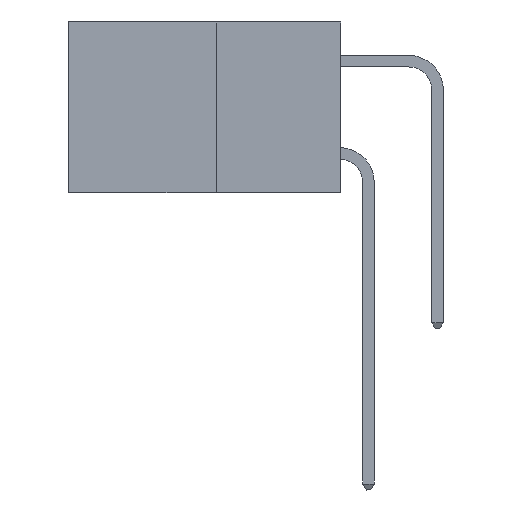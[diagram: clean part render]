
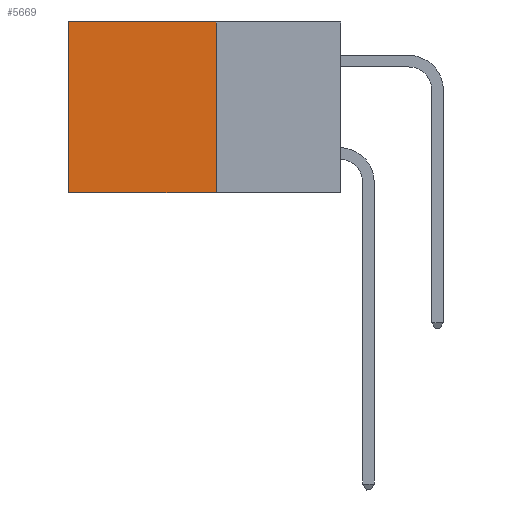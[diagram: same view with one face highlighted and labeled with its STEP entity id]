
A CAD part, left-side view. The second image highlights one B-rep face of the part: STEP entity #5669.
In plain terms, the highlighted planar face has unit normal (-1, 0, 0).
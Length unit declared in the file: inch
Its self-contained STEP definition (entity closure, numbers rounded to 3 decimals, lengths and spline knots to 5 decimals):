
#423 = EDGE_CURVE ( 'NONE', #3450, #9544, #16978, .T. ) ;
#1078 = DIRECTION ( 'NONE',  ( 0., 1., 0. ) ) ;
#1513 = EDGE_CURVE ( 'NONE', #9544, #7395, #6821, .T. ) ;
#2710 = VECTOR ( 'NONE', #7247, 39.37008 ) ;
#3160 = LINE ( 'NONE', #5839, #2710 ) ;
#3450 = VERTEX_POINT ( 'NONE', #7370 ) ;
#3506 = VECTOR ( 'NONE', #7274, 39.37008 ) ;
#4459 = CARTESIAN_POINT ( 'NONE',  ( 0.277, 0.27, -0.37 ) ) ;
#5669 = ADVANCED_FACE ( 'NONE', ( #13820 ), #6727, .F. ) ;
#5753 = VECTOR ( 'NONE', #17899, 39.37008 ) ;
#5764 = CARTESIAN_POINT ( 'NONE',  ( 0.277, 0.59, 0. ) ) ;
#5839 = CARTESIAN_POINT ( 'NONE',  ( 0.277, 0.27, -0.37 ) ) ;
#6727 = PLANE ( 'NONE',  #17481 ) ;
#6821 = LINE ( 'NONE', #13843, #3506 ) ;
#7247 = DIRECTION ( 'NONE',  ( 0., 0., -1. ) ) ;
#7274 = DIRECTION ( 'NONE',  ( 0., 0., -1. ) ) ;
#7370 = CARTESIAN_POINT ( 'NONE',  ( 0.277, 0.27, 0. ) ) ;
#7395 = VERTEX_POINT ( 'NONE', #14229 ) ;
#8131 = DIRECTION ( 'NONE',  ( 1., 0., 0. ) ) ;
#8207 = EDGE_CURVE ( 'NONE', #16064, #7395, #10710, .T. ) ;
#9095 = EDGE_LOOP ( 'NONE', ( #12071, #12832, #16765, #14040 ) ) ;
#9544 = VERTEX_POINT ( 'NONE', #5764 ) ;
#10710 = LINE ( 'NONE', #16566, #5753 ) ;
#12071 = ORIENTED_EDGE ( 'NONE', *, *, #1513, .T. ) ;
#12170 = EDGE_CURVE ( 'NONE', #3450, #16064, #3160, .T. ) ;
#12323 = CARTESIAN_POINT ( 'NONE',  ( 0.277, 0.27, 0. ) ) ;
#12832 = ORIENTED_EDGE ( 'NONE', *, *, #8207, .F. ) ;
#13820 = FACE_OUTER_BOUND ( 'NONE', #9095, .T. ) ;
#13843 = CARTESIAN_POINT ( 'NONE',  ( 0.277, 0.59, -0.37 ) ) ;
#14040 = ORIENTED_EDGE ( 'NONE', *, *, #423, .T. ) ;
#14229 = CARTESIAN_POINT ( 'NONE',  ( 0.277, 0.59, -0.37 ) ) ;
#16064 = VERTEX_POINT ( 'NONE', #4459 ) ;
#16335 = CARTESIAN_POINT ( 'NONE',  ( 0.277, 0.27, -0.37 ) ) ;
#16566 = CARTESIAN_POINT ( 'NONE',  ( 0.277, 0.27, -0.37 ) ) ;
#16580 = VECTOR ( 'NONE', #1078, 39.37008 ) ;
#16765 = ORIENTED_EDGE ( 'NONE', *, *, #12170, .F. ) ;
#16978 = LINE ( 'NONE', #12323, #16580 ) ;
#17481 = AXIS2_PLACEMENT_3D ( 'NONE', #16335, #8131, #17668 ) ;
#17668 = DIRECTION ( 'NONE',  ( 0., 0., -1. ) ) ;
#17899 = DIRECTION ( 'NONE',  ( 0., 1., 0. ) ) ;
